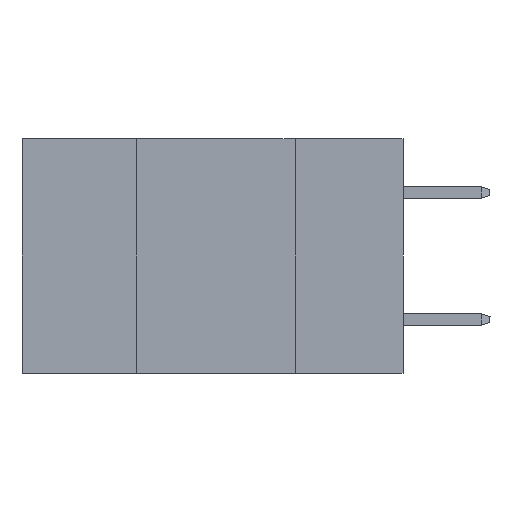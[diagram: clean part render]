
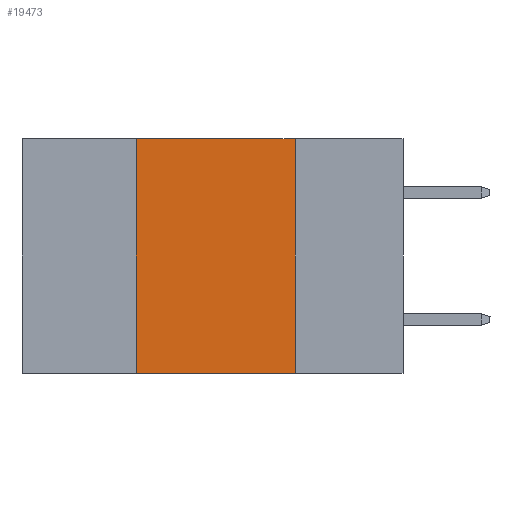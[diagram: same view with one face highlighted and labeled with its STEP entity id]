
A CAD part, left-side view. The second image highlights one B-rep face of the part: STEP entity #19473.
In plain terms, the highlighted planar face has unit normal (-1, 0, 0).
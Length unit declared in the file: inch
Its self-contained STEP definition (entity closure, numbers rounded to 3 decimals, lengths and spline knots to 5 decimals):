
#55 = LINE ( 'NONE', #10993, #10152 ) ;
#906 = VECTOR ( 'NONE', #6399, 39.37008 ) ;
#1004 = PLANE ( 'NONE',  #14514 ) ;
#1093 = EDGE_CURVE ( 'NONE', #15101, #2278, #6433, .T. ) ;
#2278 = VERTEX_POINT ( 'NONE', #17776 ) ;
#3055 = VECTOR ( 'NONE', #20117, 39.37008 ) ;
#3452 = CARTESIAN_POINT ( 'NONE',  ( 0., 0.6, 0. ) ) ;
#3891 = EDGE_CURVE ( 'NONE', #4560, #15101, #7936, .T. ) ;
#4378 = CARTESIAN_POINT ( 'NONE',  ( 0., 0.17, -0.37 ) ) ;
#4560 = VERTEX_POINT ( 'NONE', #18309 ) ;
#5760 = CARTESIAN_POINT ( 'NONE',  ( 0., 0.17, 0. ) ) ;
#6065 = ORIENTED_EDGE ( 'NONE', *, *, #1093, .F. ) ;
#6399 = DIRECTION ( 'NONE',  ( 0., 0., 1. ) ) ;
#6433 = LINE ( 'NONE', #3452, #3055 ) ;
#7936 = LINE ( 'NONE', #12809, #906 ) ;
#8680 = FACE_OUTER_BOUND ( 'NONE', #12729, .T. ) ;
#9266 = DIRECTION ( 'NONE',  ( 0., -1., 0. ) ) ;
#9439 = EDGE_CURVE ( 'NONE', #2278, #14439, #18318, .T. ) ;
#10152 = VECTOR ( 'NONE', #9266, 39.37008 ) ;
#10531 = DIRECTION ( 'NONE',  ( 0., 0., -1. ) ) ;
#10908 = ORIENTED_EDGE ( 'NONE', *, *, #15808, .T. ) ;
#10993 = CARTESIAN_POINT ( 'NONE',  ( 0., 0.6, -0.37 ) ) ;
#11324 = ORIENTED_EDGE ( 'NONE', *, *, #3891, .F. ) ;
#12729 = EDGE_LOOP ( 'NONE', ( #17740, #6065, #11324, #10908 ) ) ;
#12809 = CARTESIAN_POINT ( 'NONE',  ( 0., 0.42, 0. ) ) ;
#14439 = VERTEX_POINT ( 'NONE', #4378 ) ;
#14514 = AXIS2_PLACEMENT_3D ( 'NONE', #14907, #16639, #16542 ) ;
#14907 = CARTESIAN_POINT ( 'NONE',  ( 0., 0.6, 0. ) ) ;
#15101 = VERTEX_POINT ( 'NONE', #17707 ) ;
#15808 = EDGE_CURVE ( 'NONE', #4560, #14439, #55, .T. ) ;
#16542 = DIRECTION ( 'NONE',  ( 0., 0., -1. ) ) ;
#16639 = DIRECTION ( 'NONE',  ( 1., 0., 0. ) ) ;
#17707 = CARTESIAN_POINT ( 'NONE',  ( 0., 0.42, 0. ) ) ;
#17740 = ORIENTED_EDGE ( 'NONE', *, *, #9439, .F. ) ;
#17776 = CARTESIAN_POINT ( 'NONE',  ( 0., 0.17, 0. ) ) ;
#18309 = CARTESIAN_POINT ( 'NONE',  ( 0., 0.42, -0.37 ) ) ;
#18318 = LINE ( 'NONE', #5760, #19183 ) ;
#19183 = VECTOR ( 'NONE', #10531, 39.37008 ) ;
#19473 = ADVANCED_FACE ( 'NONE', ( #8680 ), #1004, .F. ) ;
#20117 = DIRECTION ( 'NONE',  ( 0., -1., 0. ) ) ;
